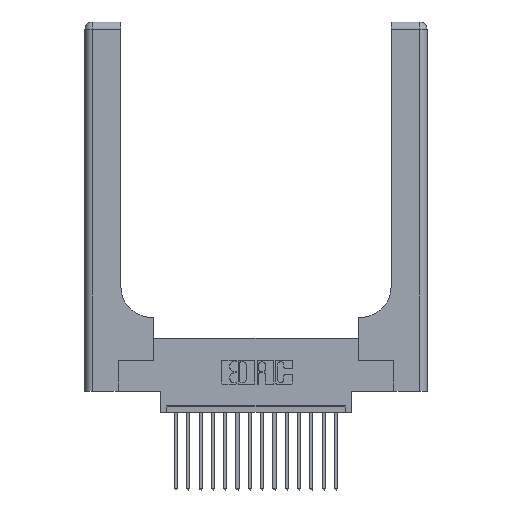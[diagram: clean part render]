
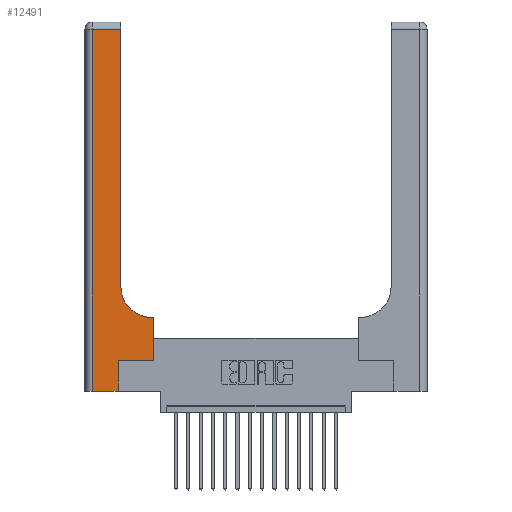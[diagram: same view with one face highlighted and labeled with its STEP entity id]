
A CAD part, top view. The second image highlights one B-rep face of the part: STEP entity #12491.
In plain terms, the highlighted planar face has unit normal (0, 0, 1).
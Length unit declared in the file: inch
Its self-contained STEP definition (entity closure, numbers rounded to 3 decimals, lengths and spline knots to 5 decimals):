
#64 = ORIENTED_EDGE ( 'NONE', *, *, #17063, .T. ) ;
#136 = VERTEX_POINT ( 'NONE', #703 ) ;
#175 = LINE ( 'NONE', #12094, #7292 ) ;
#367 = ORIENTED_EDGE ( 'NONE', *, *, #5685, .T. ) ;
#688 = CARTESIAN_POINT ( 'NONE',  ( 0.5585, 0.25, 0.37 ) ) ;
#703 = CARTESIAN_POINT ( 'NONE',  ( 0.5415, 0.6, 0.37 ) ) ;
#1028 = VECTOR ( 'NONE', #7379, 39.37008 ) ;
#1122 = VERTEX_POINT ( 'NONE', #19664 ) ;
#1577 = DIRECTION ( 'NONE',  ( 1., 0., 0. ) ) ;
#1867 = LINE ( 'NONE', #18215, #17281 ) ;
#2647 = VERTEX_POINT ( 'NONE', #18966 ) ;
#3174 = VECTOR ( 'NONE', #1577, 39.37008 ) ;
#3213 = VECTOR ( 'NONE', #11306, 39.37008 ) ;
#3626 = ORIENTED_EDGE ( 'NONE', *, *, #6223, .T. ) ;
#3674 = VERTEX_POINT ( 'NONE', #14251 ) ;
#3824 = AXIS2_PLACEMENT_3D ( 'NONE', #16872, #12074, #18247 ) ;
#4582 = VECTOR ( 'NONE', #19053, 39.37008 ) ;
#4717 = CARTESIAN_POINT ( 'NONE',  ( 0.06, 0., 0.37 ) ) ;
#4798 = CARTESIAN_POINT ( 'NONE',  ( 0.2915, 0.85, 0.37 ) ) ;
#5052 = EDGE_LOOP ( 'NONE', ( #14997, #3626, #13180, #10336, #367, #11757, #15406, #9473, #64 ) ) ;
#5054 = LINE ( 'NONE', #7524, #1028 ) ;
#5387 = CARTESIAN_POINT ( 'NONE',  ( 0., 3., 0.37 ) ) ;
#5685 = EDGE_CURVE ( 'NONE', #6967, #1122, #1867, .T. ) ;
#6136 = DIRECTION ( 'NONE',  ( 0., 1., 0. ) ) ;
#6223 = EDGE_CURVE ( 'NONE', #13533, #2647, #175, .T. ) ;
#6416 = CARTESIAN_POINT ( 'NONE',  ( 0.2915, 2.94, 0.37 ) ) ;
#6542 = VECTOR ( 'NONE', #8263, 39.37008 ) ;
#6842 = PLANE ( 'NONE',  #19655 ) ;
#6944 = CARTESIAN_POINT ( 'NONE',  ( 0.2915, 0.6, 0.37 ) ) ;
#6956 = LINE ( 'NONE', #19599, #3174 ) ;
#6967 = VERTEX_POINT ( 'NONE', #18761 ) ;
#7021 = LINE ( 'NONE', #9697, #6542 ) ;
#7035 = EDGE_CURVE ( 'NONE', #7574, #136, #16070, .T. ) ;
#7292 = VECTOR ( 'NONE', #7600, 39.37008 ) ;
#7379 = DIRECTION ( 'NONE',  ( 1., 0., 0. ) ) ;
#7416 = FACE_OUTER_BOUND ( 'NONE', #5052, .T. ) ;
#7524 = CARTESIAN_POINT ( 'NONE',  ( 0., 0., 0.37 ) ) ;
#7574 = VERTEX_POINT ( 'NONE', #14577 ) ;
#7600 = DIRECTION ( 'NONE',  ( -1., 0., 0. ) ) ;
#7685 = LINE ( 'NONE', #9870, #4582 ) ;
#8263 = DIRECTION ( 'NONE',  ( 0., 1., 0. ) ) ;
#8701 = CIRCLE ( 'NONE', #3824, 0.25 ) ;
#9038 = EDGE_CURVE ( 'NONE', #2647, #15248, #7685, .T. ) ;
#9473 = ORIENTED_EDGE ( 'NONE', *, *, #7035, .T. ) ;
#9689 = DIRECTION ( 'NONE',  ( -1., 0., 0. ) ) ;
#9697 = CARTESIAN_POINT ( 'NONE',  ( 0.2915, 3., 0.37 ) ) ;
#9870 = CARTESIAN_POINT ( 'NONE',  ( 0.06, 3., 0.37 ) ) ;
#10336 = ORIENTED_EDGE ( 'NONE', *, *, #12666, .T. ) ;
#11036 = EDGE_CURVE ( 'NONE', #3674, #7574, #16291, .T. ) ;
#11306 = DIRECTION ( 'NONE',  ( 0., 1., 0. ) ) ;
#11757 = ORIENTED_EDGE ( 'NONE', *, *, #12241, .T. ) ;
#12074 = DIRECTION ( 'NONE',  ( 0., 0., -1. ) ) ;
#12094 = CARTESIAN_POINT ( 'NONE',  ( 0., 2.94, 0.37 ) ) ;
#12232 = VECTOR ( 'NONE', #16064, 39.37008 ) ;
#12241 = EDGE_CURVE ( 'NONE', #1122, #3674, #6956, .T. ) ;
#12491 = ADVANCED_FACE ( 'NONE', ( #7416 ), #6842, .F. ) ;
#12666 = EDGE_CURVE ( 'NONE', #15248, #6967, #5054, .T. ) ;
#13009 = DIRECTION ( 'NONE',  ( 0., 0., -1. ) ) ;
#13180 = ORIENTED_EDGE ( 'NONE', *, *, #9038, .T. ) ;
#13533 = VERTEX_POINT ( 'NONE', #6416 ) ;
#14251 = CARTESIAN_POINT ( 'NONE',  ( 0.5585, 0.25, 0.37 ) ) ;
#14577 = CARTESIAN_POINT ( 'NONE',  ( 0.5585, 0.6, 0.37 ) ) ;
#14997 = ORIENTED_EDGE ( 'NONE', *, *, #19204, .T. ) ;
#15248 = VERTEX_POINT ( 'NONE', #4717 ) ;
#15406 = ORIENTED_EDGE ( 'NONE', *, *, #11036, .T. ) ;
#16064 = DIRECTION ( 'NONE',  ( -1., 0., 0. ) ) ;
#16070 = LINE ( 'NONE', #6944, #12232 ) ;
#16291 = LINE ( 'NONE', #688, #3213 ) ;
#16872 = CARTESIAN_POINT ( 'NONE',  ( 0.5415, 0.85, 0.37 ) ) ;
#17063 = EDGE_CURVE ( 'NONE', #136, #19461, #8701, .T. ) ;
#17281 = VECTOR ( 'NONE', #6136, 39.37008 ) ;
#18215 = CARTESIAN_POINT ( 'NONE',  ( 0.269, 0., 0.37 ) ) ;
#18247 = DIRECTION ( 'NONE',  ( 1., 0., 0. ) ) ;
#18761 = CARTESIAN_POINT ( 'NONE',  ( 0.269, 0., 0.37 ) ) ;
#18966 = CARTESIAN_POINT ( 'NONE',  ( 0.06, 2.94, 0.37 ) ) ;
#19053 = DIRECTION ( 'NONE',  ( 0., -1., 0. ) ) ;
#19204 = EDGE_CURVE ( 'NONE', #19461, #13533, #7021, .T. ) ;
#19461 = VERTEX_POINT ( 'NONE', #4798 ) ;
#19599 = CARTESIAN_POINT ( 'NONE',  ( 0.269, 0.25, 0.37 ) ) ;
#19655 = AXIS2_PLACEMENT_3D ( 'NONE', #5387, #13009, #9689 ) ;
#19664 = CARTESIAN_POINT ( 'NONE',  ( 0.269, 0.25, 0.37 ) ) ;
